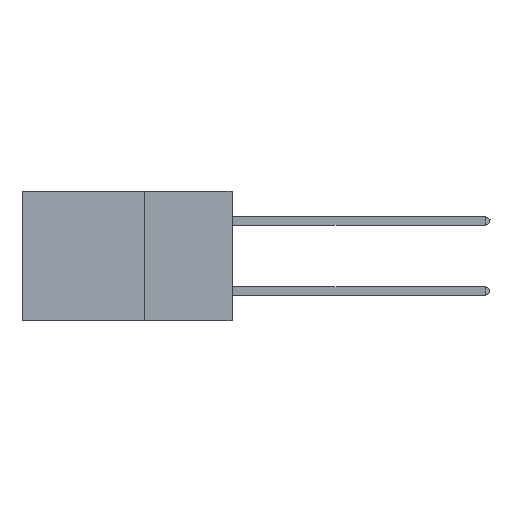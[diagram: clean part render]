
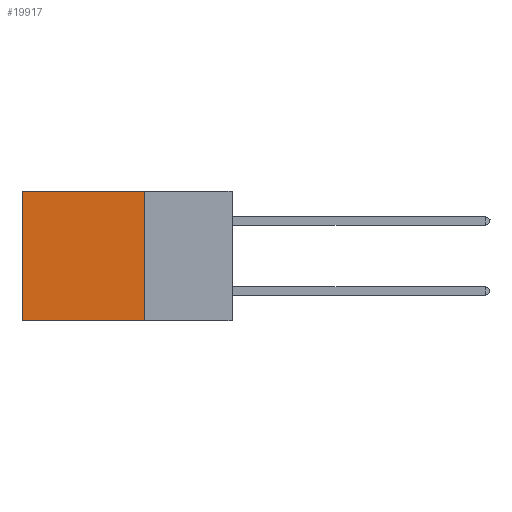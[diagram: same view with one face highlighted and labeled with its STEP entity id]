
A CAD part, left-side view. The second image highlights one B-rep face of the part: STEP entity #19917.
In plain terms, the highlighted planar face has unit normal (-1, 0, 0).
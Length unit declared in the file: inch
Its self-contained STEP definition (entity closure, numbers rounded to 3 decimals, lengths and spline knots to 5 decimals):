
#100 = VERTEX_POINT ( 'NONE', #23429 ) ;
#120 = DIRECTION ( 'NONE',  ( 1., 0., 0. ) ) ;
#594 = FACE_OUTER_BOUND ( 'NONE', #23103, .T. ) ;
#805 = VERTEX_POINT ( 'NONE', #18632 ) ;
#1195 = ORIENTED_EDGE ( 'NONE', *, *, #26205, .F. ) ;
#1845 = LINE ( 'NONE', #12712, #23741 ) ;
#2373 = AXIS2_PLACEMENT_3D ( 'NONE', #12869, #120, #21593 ) ;
#3365 = CARTESIAN_POINT ( 'NONE',  ( 0.2875, 0.25, -0.37 ) ) ;
#3479 = ORIENTED_EDGE ( 'NONE', *, *, #21877, .T. ) ;
#5425 = CARTESIAN_POINT ( 'NONE',  ( 0.2875, 0.25, 0. ) ) ;
#6619 = LINE ( 'NONE', #3365, #11995 ) ;
#6698 = PLANE ( 'NONE',  #2373 ) ;
#9904 = DIRECTION ( 'NONE',  ( 0., 0., -1. ) ) ;
#10290 = LINE ( 'NONE', #5425, #22603 ) ;
#11108 = LINE ( 'NONE', #26288, #21129 ) ;
#11995 = VECTOR ( 'NONE', #22400, 39.37008 ) ;
#12712 = CARTESIAN_POINT ( 'NONE',  ( 0.2875, 0.25, 0. ) ) ;
#12750 = VERTEX_POINT ( 'NONE', #26179 ) ;
#12869 = CARTESIAN_POINT ( 'NONE',  ( 0.2875, 0.25, 0. ) ) ;
#14585 = ORIENTED_EDGE ( 'NONE', *, *, #15236, .T. ) ;
#15236 = EDGE_CURVE ( 'NONE', #100, #12750, #11108, .T. ) ;
#16721 = DIRECTION ( 'NONE',  ( 0., 1., 0. ) ) ;
#18344 = EDGE_CURVE ( 'NONE', #26121, #805, #10290, .T. ) ;
#18632 = CARTESIAN_POINT ( 'NONE',  ( 0.2875, 0.25, -0.37 ) ) ;
#19746 = CARTESIAN_POINT ( 'NONE',  ( 0.2875, 0.25, 0. ) ) ;
#19917 = ADVANCED_FACE ( 'NONE', ( #594 ), #6698, .F. ) ;
#20789 = ORIENTED_EDGE ( 'NONE', *, *, #18344, .F. ) ;
#21129 = VECTOR ( 'NONE', #24263, 39.37008 ) ;
#21593 = DIRECTION ( 'NONE',  ( 0., 0., -1. ) ) ;
#21877 = EDGE_CURVE ( 'NONE', #26121, #100, #1845, .T. ) ;
#22400 = DIRECTION ( 'NONE',  ( 0., 1., 0. ) ) ;
#22603 = VECTOR ( 'NONE', #9904, 39.37008 ) ;
#23103 = EDGE_LOOP ( 'NONE', ( #14585, #1195, #20789, #3479 ) ) ;
#23429 = CARTESIAN_POINT ( 'NONE',  ( 0.2875, 0.6, 0. ) ) ;
#23741 = VECTOR ( 'NONE', #16721, 39.37008 ) ;
#24263 = DIRECTION ( 'NONE',  ( 0., 0., -1. ) ) ;
#26121 = VERTEX_POINT ( 'NONE', #19746 ) ;
#26179 = CARTESIAN_POINT ( 'NONE',  ( 0.2875, 0.6, -0.37 ) ) ;
#26205 = EDGE_CURVE ( 'NONE', #805, #12750, #6619, .T. ) ;
#26288 = CARTESIAN_POINT ( 'NONE',  ( 0.2875, 0.6, 0. ) ) ;
